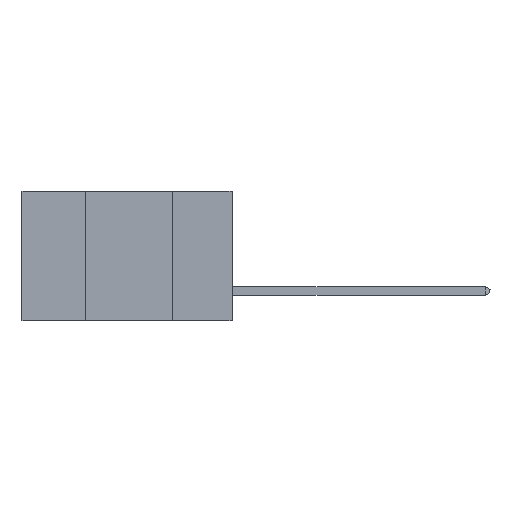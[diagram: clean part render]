
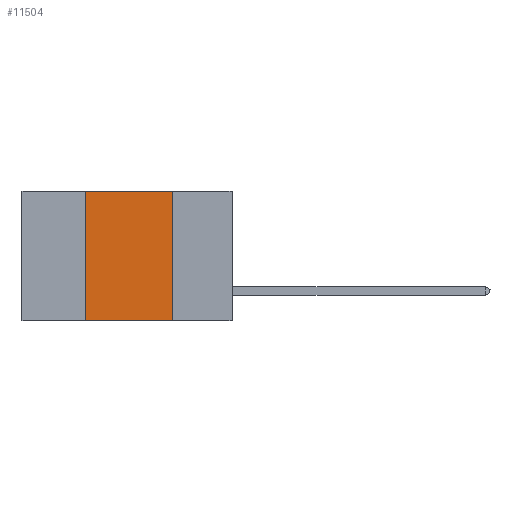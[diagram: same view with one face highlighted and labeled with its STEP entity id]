
A CAD part, left-side view. The second image highlights one B-rep face of the part: STEP entity #11504.
In plain terms, the highlighted planar face has unit normal (-1, 0, 0).
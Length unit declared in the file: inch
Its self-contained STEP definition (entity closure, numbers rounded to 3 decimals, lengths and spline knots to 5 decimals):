
#170 = CARTESIAN_POINT ( 'NONE',  ( 0., 0.42, 0. ) ) ;
#199 = EDGE_CURVE ( 'NONE', #11163, #9942, #488, .T. ) ;
#320 = VECTOR ( 'NONE', #6811, 39.37008 ) ;
#448 = ORIENTED_EDGE ( 'NONE', *, *, #10210, .F. ) ;
#488 = LINE ( 'NONE', #10087, #320 ) ;
#1353 = FACE_OUTER_BOUND ( 'NONE', #2366, .T. ) ;
#1543 = EDGE_CURVE ( 'NONE', #11476, #7810, #2627, .T. ) ;
#1860 = CARTESIAN_POINT ( 'NONE',  ( 0., 0.17, -0.37 ) ) ;
#2366 = EDGE_LOOP ( 'NONE', ( #448, #4532, #4707, #9218 ) ) ;
#2627 = LINE ( 'NONE', #2971, #10805 ) ;
#2853 = LINE ( 'NONE', #170, #8188 ) ;
#2971 = CARTESIAN_POINT ( 'NONE',  ( 0., 0.6, -0.37 ) ) ;
#3252 = LINE ( 'NONE', #11430, #8405 ) ;
#3681 = DIRECTION ( 'NONE',  ( 1., 0., 0. ) ) ;
#3727 = CARTESIAN_POINT ( 'NONE',  ( 0., 0.6, 0. ) ) ;
#3730 = CARTESIAN_POINT ( 'NONE',  ( 0., 0.42, 0. ) ) ;
#4532 = ORIENTED_EDGE ( 'NONE', *, *, #199, .F. ) ;
#4707 = ORIENTED_EDGE ( 'NONE', *, *, #5975, .F. ) ;
#4885 = DIRECTION ( 'NONE',  ( 0., 0., -1. ) ) ;
#5975 = EDGE_CURVE ( 'NONE', #11476, #11163, #2853, .T. ) ;
#6811 = DIRECTION ( 'NONE',  ( 0., -1., 0. ) ) ;
#7810 = VERTEX_POINT ( 'NONE', #1860 ) ;
#8050 = AXIS2_PLACEMENT_3D ( 'NONE', #3727, #3681, #4885 ) ;
#8187 = DIRECTION ( 'NONE',  ( 0., -1., 0. ) ) ;
#8188 = VECTOR ( 'NONE', #9545, 39.37008 ) ;
#8405 = VECTOR ( 'NONE', #12352, 39.37008 ) ;
#9218 = ORIENTED_EDGE ( 'NONE', *, *, #1543, .T. ) ;
#9545 = DIRECTION ( 'NONE',  ( 0., 0., 1. ) ) ;
#9942 = VERTEX_POINT ( 'NONE', #11903 ) ;
#10048 = PLANE ( 'NONE',  #8050 ) ;
#10087 = CARTESIAN_POINT ( 'NONE',  ( 0., 0.6, 0. ) ) ;
#10210 = EDGE_CURVE ( 'NONE', #9942, #7810, #3252, .T. ) ;
#10805 = VECTOR ( 'NONE', #8187, 39.37008 ) ;
#11163 = VERTEX_POINT ( 'NONE', #3730 ) ;
#11169 = CARTESIAN_POINT ( 'NONE',  ( 0., 0.42, -0.37 ) ) ;
#11430 = CARTESIAN_POINT ( 'NONE',  ( 0., 0.17, 0. ) ) ;
#11476 = VERTEX_POINT ( 'NONE', #11169 ) ;
#11504 = ADVANCED_FACE ( 'NONE', ( #1353 ), #10048, .F. ) ;
#11903 = CARTESIAN_POINT ( 'NONE',  ( 0., 0.17, 0. ) ) ;
#12352 = DIRECTION ( 'NONE',  ( 0., 0., -1. ) ) ;
